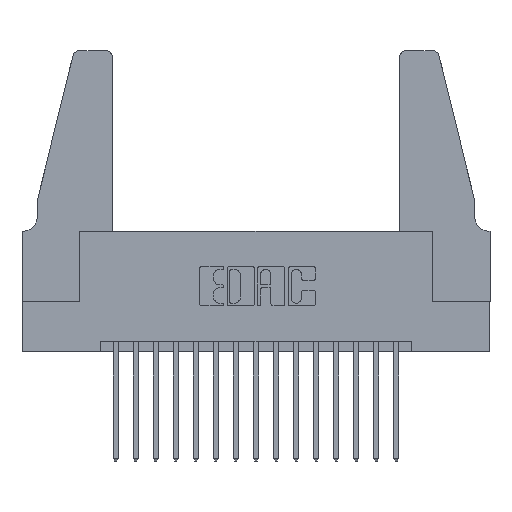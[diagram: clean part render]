
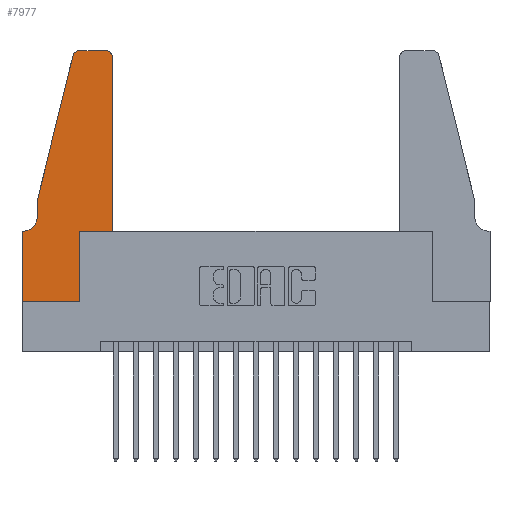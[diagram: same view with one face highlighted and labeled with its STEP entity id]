
A CAD part, top view. The second image highlights one B-rep face of the part: STEP entity #7977.
In plain terms, the highlighted planar face has unit normal (0, 0, 1).
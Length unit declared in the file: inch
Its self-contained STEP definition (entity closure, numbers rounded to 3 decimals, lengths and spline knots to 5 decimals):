
#114 = ORIENTED_EDGE ( 'NONE', *, *, #16000, .T. ) ;
#616 = VERTEX_POINT ( 'NONE', #799 ) ;
#773 = CARTESIAN_POINT ( 'NONE',  ( 0.4205, 1.25, 0.37 ) ) ;
#799 = CARTESIAN_POINT ( 'NONE',  ( 0., 0.35, 0.37 ) ) ;
#847 = EDGE_CURVE ( 'NONE', #5193, #15640, #14827, .T. ) ;
#1245 = CARTESIAN_POINT ( 'NONE',  ( 0.4505, 0.35, 0.37 ) ) ;
#1268 = CARTESIAN_POINT ( 'NONE',  ( 0.0755, 0.5, 0.37 ) ) ;
#1271 = VERTEX_POINT ( 'NONE', #17318 ) ;
#1616 = EDGE_CURVE ( 'NONE', #6257, #11793, #4805, .T. ) ;
#1735 = CARTESIAN_POINT ( 'NONE',  ( 0.2605, 1.25, 0.37 ) ) ;
#1739 = VECTOR ( 'NONE', #8867, 39.37008 ) ;
#1879 = EDGE_CURVE ( 'NONE', #616, #14310, #9764, .T. ) ;
#2540 = FACE_OUTER_BOUND ( 'NONE', #7058, .T. ) ;
#2572 = CIRCLE ( 'NONE', #6907, 0.07 ) ;
#2721 = VECTOR ( 'NONE', #5822, 39.37008 ) ;
#3000 = ORIENTED_EDGE ( 'NONE', *, *, #6999, .T. ) ;
#3023 = ORIENTED_EDGE ( 'NONE', *, *, #5180, .T. ) ;
#3626 = ORIENTED_EDGE ( 'NONE', *, *, #15937, .T. ) ;
#3641 = VECTOR ( 'NONE', #5899, 39.37008 ) ;
#3972 = ORIENTED_EDGE ( 'NONE', *, *, #12434, .T. ) ;
#4084 = LINE ( 'NONE', #13817, #16168 ) ;
#4196 = VECTOR ( 'NONE', #13265, 39.37008 ) ;
#4268 = VERTEX_POINT ( 'NONE', #16187 ) ;
#4503 = VERTEX_POINT ( 'NONE', #10818 ) ;
#4597 = DIRECTION ( 'NONE',  ( 0., 0., -1. ) ) ;
#4805 = LINE ( 'NONE', #1268, #4196 ) ;
#4979 = CARTESIAN_POINT ( 'NONE',  ( 0., 0., 0.37 ) ) ;
#4983 = DIRECTION ( 'NONE',  ( 0., 0., 1. ) ) ;
#5180 = EDGE_CURVE ( 'NONE', #15640, #7799, #11370, .T. ) ;
#5193 = VERTEX_POINT ( 'NONE', #773 ) ;
#5602 = VECTOR ( 'NONE', #10201, 39.37008 ) ;
#5632 = DIRECTION ( 'NONE',  ( 1., 0., 0. ) ) ;
#5793 = CARTESIAN_POINT ( 'NONE',  ( 0.25487, 1.22718, 0.37 ) ) ;
#5822 = DIRECTION ( 'NONE',  ( -1., 0., 0. ) ) ;
#5874 = VERTEX_POINT ( 'NONE', #16878 ) ;
#5899 = DIRECTION ( 'NONE',  ( 1., 0., 0. ) ) ;
#6164 = CARTESIAN_POINT ( 'NONE',  ( 0.0755, 0.5, 0.37 ) ) ;
#6257 = VERTEX_POINT ( 'NONE', #7043 ) ;
#6404 = LINE ( 'NONE', #1245, #15527 ) ;
#6907 = AXIS2_PLACEMENT_3D ( 'NONE', #8448, #4597, #8757 ) ;
#6999 = EDGE_CURVE ( 'NONE', #7799, #6257, #13406, .T. ) ;
#7043 = CARTESIAN_POINT ( 'NONE',  ( 0.0755, 0.5, 0.37 ) ) ;
#7058 = EDGE_LOOP ( 'NONE', ( #15715, #3023, #3000, #12735, #8888, #15112, #14209, #114, #11787, #3972, #3626, #7974 ) ) ;
#7302 = EDGE_CURVE ( 'NONE', #4268, #5193, #16978, .T. ) ;
#7713 = LINE ( 'NONE', #12847, #5602 ) ;
#7799 = VERTEX_POINT ( 'NONE', #5793 ) ;
#7974 = ORIENTED_EDGE ( 'NONE', *, *, #7302, .T. ) ;
#7977 = ADVANCED_FACE ( 'NONE', ( #2540 ), #13640, .T. ) ;
#8046 = DIRECTION ( 'NONE',  ( 0., 0., 1. ) ) ;
#8164 = CARTESIAN_POINT ( 'NONE',  ( 0.4205, 1.22, 0.37 ) ) ;
#8336 = CARTESIAN_POINT ( 'NONE',  ( 0.0755, 0.42, 0.37 ) ) ;
#8448 = CARTESIAN_POINT ( 'NONE',  ( 0.0055, 0.42, 0.37 ) ) ;
#8565 = VERTEX_POINT ( 'NONE', #12304 ) ;
#8616 = CARTESIAN_POINT ( 'NONE',  ( 0.2865, 0.35, 0.37 ) ) ;
#8757 = DIRECTION ( 'NONE',  ( -1., 0., 0. ) ) ;
#8867 = DIRECTION ( 'NONE',  ( -0.239, -0.971, 0. ) ) ;
#8888 = ORIENTED_EDGE ( 'NONE', *, *, #17356, .T. ) ;
#9724 = CARTESIAN_POINT ( 'NONE',  ( 0.4505, 0.35, 0.37 ) ) ;
#9764 = LINE ( 'NONE', #11144, #12706 ) ;
#10201 = DIRECTION ( 'NONE',  ( -1., 0., 0. ) ) ;
#10818 = CARTESIAN_POINT ( 'NONE',  ( 0.2865, 0., 0.37 ) ) ;
#11144 = CARTESIAN_POINT ( 'NONE',  ( 0., 0., 0.37 ) ) ;
#11155 = AXIS2_PLACEMENT_3D ( 'NONE', #13803, #16407, #5632 ) ;
#11234 = DIRECTION ( 'NONE',  ( 1., 0., 0. ) ) ;
#11344 = DIRECTION ( 'NONE',  ( 0., 1., 0. ) ) ;
#11370 = CIRCLE ( 'NONE', #17571, 0.03 ) ;
#11683 = EDGE_CURVE ( 'NONE', #5874, #616, #7713, .T. ) ;
#11787 = ORIENTED_EDGE ( 'NONE', *, *, #16117, .T. ) ;
#11793 = VERTEX_POINT ( 'NONE', #8336 ) ;
#12196 = DIRECTION ( 'NONE',  ( 0., 1., 0. ) ) ;
#12304 = CARTESIAN_POINT ( 'NONE',  ( 0.2865, 0.35, 0.37 ) ) ;
#12434 = EDGE_CURVE ( 'NONE', #8565, #1271, #17422, .T. ) ;
#12706 = VECTOR ( 'NONE', #13834, 39.37008 ) ;
#12735 = ORIENTED_EDGE ( 'NONE', *, *, #1616, .T. ) ;
#12847 = CARTESIAN_POINT ( 'NONE',  ( 0.0755, 0.35, 0.37 ) ) ;
#13004 = LINE ( 'NONE', #8616, #16785 ) ;
#13265 = DIRECTION ( 'NONE',  ( 0., -1., 0. ) ) ;
#13406 = LINE ( 'NONE', #6164, #1739 ) ;
#13640 = PLANE ( 'NONE',  #11155 ) ;
#13729 = AXIS2_PLACEMENT_3D ( 'NONE', #8164, #8046, #14913 ) ;
#13803 = CARTESIAN_POINT ( 'NONE',  ( 0., 0.35, 0.37 ) ) ;
#13817 = CARTESIAN_POINT ( 'NONE',  ( 0., 0., 0.37 ) ) ;
#13834 = DIRECTION ( 'NONE',  ( 0., -1., 0. ) ) ;
#14209 = ORIENTED_EDGE ( 'NONE', *, *, #1879, .T. ) ;
#14286 = DIRECTION ( 'NONE',  ( 1., 0., 0. ) ) ;
#14310 = VERTEX_POINT ( 'NONE', #4979 ) ;
#14422 = CARTESIAN_POINT ( 'NONE',  ( 0.284, 1.25, 0.37 ) ) ;
#14827 = LINE ( 'NONE', #1735, #2721 ) ;
#14913 = DIRECTION ( 'NONE',  ( 1., 0., 0. ) ) ;
#15112 = ORIENTED_EDGE ( 'NONE', *, *, #11683, .T. ) ;
#15527 = VECTOR ( 'NONE', #12196, 39.37008 ) ;
#15640 = VERTEX_POINT ( 'NONE', #14422 ) ;
#15715 = ORIENTED_EDGE ( 'NONE', *, *, #847, .T. ) ;
#15937 = EDGE_CURVE ( 'NONE', #1271, #4268, #6404, .T. ) ;
#16000 = EDGE_CURVE ( 'NONE', #14310, #4503, #4084, .T. ) ;
#16117 = EDGE_CURVE ( 'NONE', #4503, #8565, #13004, .T. ) ;
#16168 = VECTOR ( 'NONE', #11234, 39.37008 ) ;
#16187 = CARTESIAN_POINT ( 'NONE',  ( 0.4505, 1.22, 0.37 ) ) ;
#16407 = DIRECTION ( 'NONE',  ( 0., 0., 1. ) ) ;
#16785 = VECTOR ( 'NONE', #11344, 39.37008 ) ;
#16878 = CARTESIAN_POINT ( 'NONE',  ( 0.0055, 0.35, 0.37 ) ) ;
#16978 = CIRCLE ( 'NONE', #13729, 0.03 ) ;
#17132 = CARTESIAN_POINT ( 'NONE',  ( 0.284, 1.22, 0.37 ) ) ;
#17318 = CARTESIAN_POINT ( 'NONE',  ( 0.4505, 0.35, 0.37 ) ) ;
#17356 = EDGE_CURVE ( 'NONE', #11793, #5874, #2572, .T. ) ;
#17422 = LINE ( 'NONE', #9724, #3641 ) ;
#17571 = AXIS2_PLACEMENT_3D ( 'NONE', #17132, #4983, #14286 ) ;
